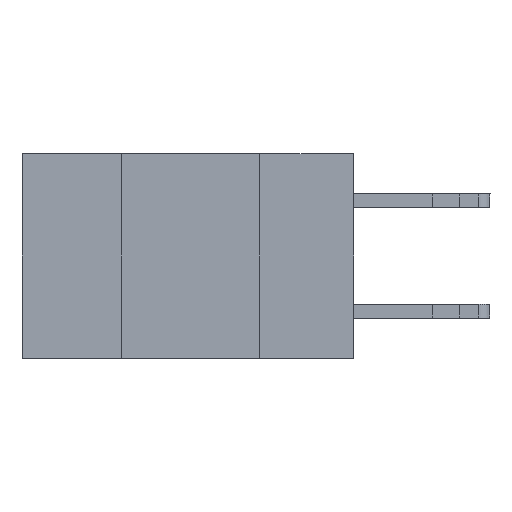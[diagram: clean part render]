
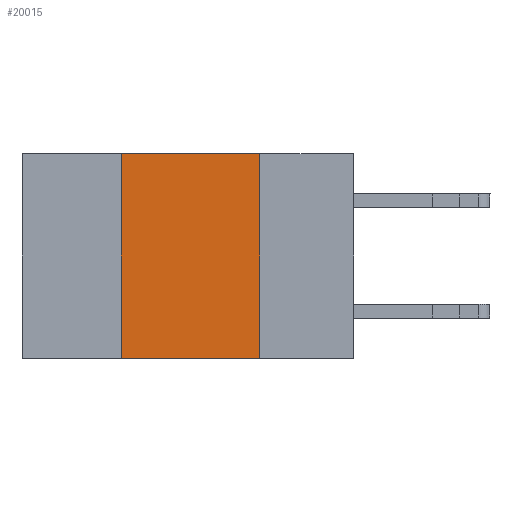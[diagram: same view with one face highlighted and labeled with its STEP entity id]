
A CAD part, left-side view. The second image highlights one B-rep face of the part: STEP entity #20015.
In plain terms, the highlighted planar face has unit normal (-1, 0, 0).
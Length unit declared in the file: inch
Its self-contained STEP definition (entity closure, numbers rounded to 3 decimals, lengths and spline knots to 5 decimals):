
#233 = ORIENTED_EDGE ( 'NONE', *, *, #13851, .F. ) ;
#2121 = DIRECTION ( 'NONE',  ( 0., 0., -1. ) ) ;
#3509 = DIRECTION ( 'NONE',  ( 0., 0., 1. ) ) ;
#3889 = AXIS2_PLACEMENT_3D ( 'NONE', #20554, #9376, #18554 ) ;
#4069 = PLANE ( 'NONE',  #3889 ) ;
#5313 = CARTESIAN_POINT ( 'NONE',  ( 0., 0.42, 0. ) ) ;
#6180 = EDGE_LOOP ( 'NONE', ( #14671, #9428, #233, #13674 ) ) ;
#7471 = VERTEX_POINT ( 'NONE', #19313 ) ;
#8022 = LINE ( 'NONE', #14538, #13223 ) ;
#8502 = VERTEX_POINT ( 'NONE', #15826 ) ;
#9376 = DIRECTION ( 'NONE',  ( 1., 0., 0. ) ) ;
#9428 = ORIENTED_EDGE ( 'NONE', *, *, #20800, .F. ) ;
#11177 = VERTEX_POINT ( 'NONE', #5313 ) ;
#11185 = VERTEX_POINT ( 'NONE', #16574 ) ;
#11334 = DIRECTION ( 'NONE',  ( 0., -1., 0. ) ) ;
#11445 = CARTESIAN_POINT ( 'NONE',  ( 0., 0.17, 0. ) ) ;
#11820 = DIRECTION ( 'NONE',  ( 0., -1., 0. ) ) ;
#12946 = VECTOR ( 'NONE', #11334, 39.37008 ) ;
#13223 = VECTOR ( 'NONE', #3509, 39.37008 ) ;
#13674 = ORIENTED_EDGE ( 'NONE', *, *, #23748, .T. ) ;
#13851 = EDGE_CURVE ( 'NONE', #11185, #11177, #8022, .T. ) ;
#14538 = CARTESIAN_POINT ( 'NONE',  ( 0., 0.42, 0. ) ) ;
#14671 = ORIENTED_EDGE ( 'NONE', *, *, #22237, .F. ) ;
#15826 = CARTESIAN_POINT ( 'NONE',  ( 0., 0.17, 0. ) ) ;
#16574 = CARTESIAN_POINT ( 'NONE',  ( 0., 0.42, -0.37 ) ) ;
#17681 = LINE ( 'NONE', #21151, #23129 ) ;
#18554 = DIRECTION ( 'NONE',  ( 0., 0., -1. ) ) ;
#19313 = CARTESIAN_POINT ( 'NONE',  ( 0., 0.17, -0.37 ) ) ;
#19461 = VECTOR ( 'NONE', #2121, 39.37008 ) ;
#19566 = LINE ( 'NONE', #22161, #12946 ) ;
#20015 = ADVANCED_FACE ( 'NONE', ( #23567 ), #4069, .F. ) ;
#20554 = CARTESIAN_POINT ( 'NONE',  ( 0., 0.6, 0. ) ) ;
#20800 = EDGE_CURVE ( 'NONE', #11177, #8502, #19566, .T. ) ;
#20897 = LINE ( 'NONE', #11445, #19461 ) ;
#21151 = CARTESIAN_POINT ( 'NONE',  ( 0., 0.6, -0.37 ) ) ;
#22161 = CARTESIAN_POINT ( 'NONE',  ( 0., 0.6, 0. ) ) ;
#22237 = EDGE_CURVE ( 'NONE', #8502, #7471, #20897, .T. ) ;
#23129 = VECTOR ( 'NONE', #11820, 39.37008 ) ;
#23567 = FACE_OUTER_BOUND ( 'NONE', #6180, .T. ) ;
#23748 = EDGE_CURVE ( 'NONE', #11185, #7471, #17681, .T. ) ;
